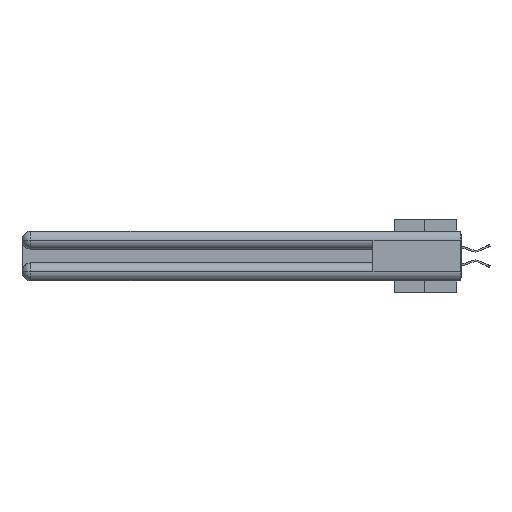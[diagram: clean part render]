
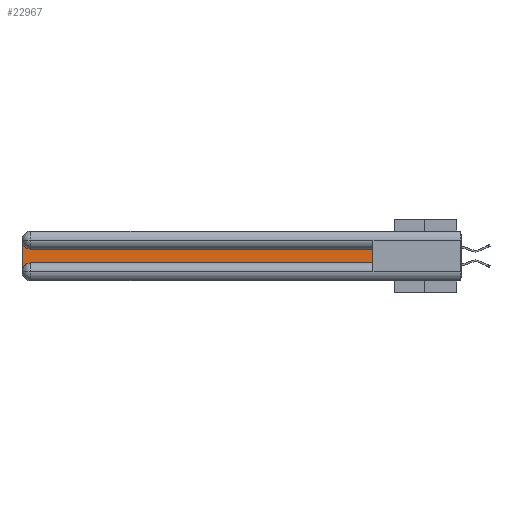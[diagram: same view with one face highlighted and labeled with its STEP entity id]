
A CAD part, left-side view. The second image highlights one B-rep face of the part: STEP entity #22967.
In plain terms, the highlighted planar face has unit normal (-1, 0, 0).
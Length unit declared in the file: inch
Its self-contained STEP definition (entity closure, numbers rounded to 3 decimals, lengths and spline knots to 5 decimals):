
#86 = CARTESIAN_POINT ( 'NONE',  ( 0.075, 0.6, -0.2175 ) ) ;
#363 = CARTESIAN_POINT ( 'NONE',  ( 0.075, 2.94, -0.2775 ) ) ;
#469 = CARTESIAN_POINT ( 'NONE',  ( 0.075, 3., -0.1225 ) ) ;
#648 = ORIENTED_EDGE ( 'NONE', *, *, #32357, .T. ) ;
#853 = DIRECTION ( 'NONE',  ( 1., 0., 0. ) ) ;
#1476 = LINE ( 'NONE', #23714, #27849 ) ;
#2842 = CARTESIAN_POINT ( 'NONE',  ( 0.075, 2.94, -0.2175 ) ) ;
#3522 = DIRECTION ( 'NONE',  ( 0., 0., -1. ) ) ;
#3726 = AXIS2_PLACEMENT_3D ( 'NONE', #7959, #5301, #7823 ) ;
#5301 = DIRECTION ( 'NONE',  ( 1., 0., 0. ) ) ;
#5510 = VERTEX_POINT ( 'NONE', #13354 ) ;
#6067 = FACE_OUTER_BOUND ( 'NONE', #24096, .T. ) ;
#6478 = DIRECTION ( 'NONE',  ( 1., 0., 0. ) ) ;
#6756 = VECTOR ( 'NONE', #37559, 39.37008 ) ;
#7778 = CIRCLE ( 'NONE', #3726, 0.06 ) ;
#7823 = DIRECTION ( 'NONE',  ( 0., 0., -1. ) ) ;
#7959 = CARTESIAN_POINT ( 'NONE',  ( 0.075, 2.94, -0.0625 ) ) ;
#11494 = VERTEX_POINT ( 'NONE', #2842 ) ;
#12074 = PLANE ( 'NONE',  #13204 ) ;
#13204 = AXIS2_PLACEMENT_3D ( 'NONE', #469, #853, #23869 ) ;
#13244 = EDGE_CURVE ( 'NONE', #27553, #30571, #33402, .T. ) ;
#13354 = CARTESIAN_POINT ( 'NONE',  ( 0.075, 3., -0.2775 ) ) ;
#14271 = VECTOR ( 'NONE', #28051, 39.37008 ) ;
#14338 = ORIENTED_EDGE ( 'NONE', *, *, #30644, .T. ) ;
#14468 = LINE ( 'NONE', #86, #6756 ) ;
#15108 = ORIENTED_EDGE ( 'NONE', *, *, #13244, .T. ) ;
#15501 = EDGE_CURVE ( 'NONE', #5510, #11494, #27707, .T. ) ;
#16909 = ORIENTED_EDGE ( 'NONE', *, *, #20171, .T. ) ;
#17125 = CARTESIAN_POINT ( 'NONE',  ( 0.075, 2.94, -0.1225 ) ) ;
#17455 = CARTESIAN_POINT ( 'NONE',  ( 0.075, 0.6, -0.2175 ) ) ;
#17546 = CARTESIAN_POINT ( 'NONE',  ( 0.075, 3., -0.0625 ) ) ;
#20171 = EDGE_CURVE ( 'NONE', #30571, #29880, #7778, .T. ) ;
#20976 = CARTESIAN_POINT ( 'NONE',  ( 0.075, 0.6, -0.2175 ) ) ;
#22168 = CARTESIAN_POINT ( 'NONE',  ( 0.075, 0.6, -0.1225 ) ) ;
#22967 = ADVANCED_FACE ( 'NONE', ( #6067 ), #12074, .F. ) ;
#23714 = CARTESIAN_POINT ( 'NONE',  ( 0.075, 3., -0.2175 ) ) ;
#23869 = DIRECTION ( 'NONE',  ( 0., 0., -1. ) ) ;
#24096 = EDGE_LOOP ( 'NONE', ( #15108, #16909, #648, #36581, #14338, #27026 ) ) ;
#27026 = ORIENTED_EDGE ( 'NONE', *, *, #31258, .T. ) ;
#27553 = VERTEX_POINT ( 'NONE', #28765 ) ;
#27616 = LINE ( 'NONE', #17455, #35888 ) ;
#27707 = CIRCLE ( 'NONE', #33091, 0.06 ) ;
#27849 = VECTOR ( 'NONE', #37779, 39.37008 ) ;
#28051 = DIRECTION ( 'NONE',  ( 0., 1., 0. ) ) ;
#28765 = CARTESIAN_POINT ( 'NONE',  ( 0.075, 0.6, -0.1225 ) ) ;
#29314 = DIRECTION ( 'NONE',  ( 0., 0., 1. ) ) ;
#29880 = VERTEX_POINT ( 'NONE', #17546 ) ;
#30571 = VERTEX_POINT ( 'NONE', #17125 ) ;
#30644 = EDGE_CURVE ( 'NONE', #11494, #36188, #14468, .T. ) ;
#31258 = EDGE_CURVE ( 'NONE', #36188, #27553, #27616, .T. ) ;
#32357 = EDGE_CURVE ( 'NONE', #29880, #5510, #1476, .T. ) ;
#33091 = AXIS2_PLACEMENT_3D ( 'NONE', #363, #6478, #3522 ) ;
#33402 = LINE ( 'NONE', #22168, #14271 ) ;
#35888 = VECTOR ( 'NONE', #29314, 39.37008 ) ;
#36188 = VERTEX_POINT ( 'NONE', #20976 ) ;
#36581 = ORIENTED_EDGE ( 'NONE', *, *, #15501, .T. ) ;
#37559 = DIRECTION ( 'NONE',  ( 0., -1., 0. ) ) ;
#37779 = DIRECTION ( 'NONE',  ( 0., 0., -1. ) ) ;
